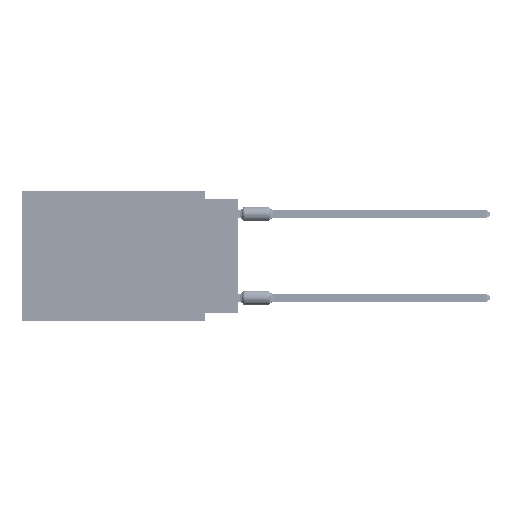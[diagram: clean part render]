
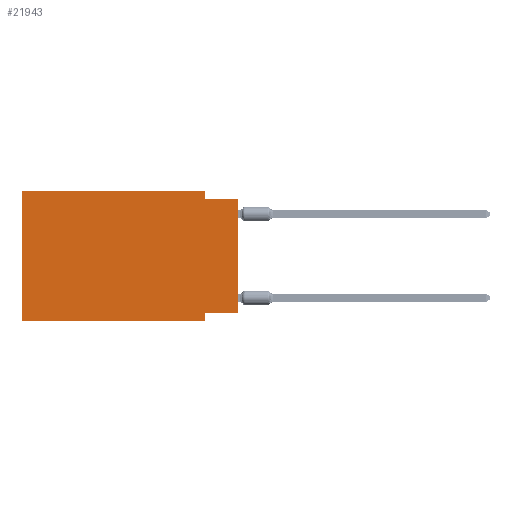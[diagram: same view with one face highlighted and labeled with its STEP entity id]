
A CAD part, left-side view. The second image highlights one B-rep face of the part: STEP entity #21943.
In plain terms, the highlighted planar face has unit normal (-1, 0, 0).
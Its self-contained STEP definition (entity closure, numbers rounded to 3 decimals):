
#1484 = LINE ( 'NONE', #72477, #11325 ) ;
#3203 = DIRECTION ( 'NONE',  ( 0., 0., 1. ) ) ;
#3818 = CARTESIAN_POINT ( 'NONE',  ( 0., 2.54, -9.271 ) ) ;
#4846 = VECTOR ( 'NONE', #40684, 1000. ) ;
#6662 = EDGE_LOOP ( 'NONE', ( #53667, #39461, #34079, #17401, #43383, #15683, #40412, #62274 ) ) ;
#9357 = DIRECTION ( 'NONE',  ( 0., -1., 0. ) ) ;
#11148 = EDGE_CURVE ( 'NONE', #65817, #14942, #81049, .T. ) ;
#11244 = VERTEX_POINT ( 'NONE', #76825 ) ;
#11325 = VECTOR ( 'NONE', #66577, 1000. ) ;
#13770 = CARTESIAN_POINT ( 'NONE',  ( 0., 16.383, 0. ) ) ;
#13896 = VERTEX_POINT ( 'NONE', #51735 ) ;
#14942 = VERTEX_POINT ( 'NONE', #24481 ) ;
#15283 = AXIS2_PLACEMENT_3D ( 'NONE', #20188, #45797, #71420 ) ;
#15683 = ORIENTED_EDGE ( 'NONE', *, *, #73483, .T. ) ;
#16409 = CARTESIAN_POINT ( 'NONE',  ( 0., 16.383, -9.906 ) ) ;
#16473 = CARTESIAN_POINT ( 'NONE',  ( 0., 0., -0.635 ) ) ;
#17401 = ORIENTED_EDGE ( 'NONE', *, *, #70530, .F. ) ;
#18033 = CARTESIAN_POINT ( 'NONE',  ( 0., 2.54, 0. ) ) ;
#18951 = FACE_OUTER_BOUND ( 'NONE', #6662, .T. ) ;
#20103 = VECTOR ( 'NONE', #43658, 1000. ) ;
#20188 = CARTESIAN_POINT ( 'NONE',  ( 0., 16.383, 0. ) ) ;
#21943 = ADVANCED_FACE ( 'NONE', ( #18951 ), #26496, .F. ) ;
#24481 = CARTESIAN_POINT ( 'NONE',  ( 0., 2.54, -0.635 ) ) ;
#24612 = VERTEX_POINT ( 'NONE', #16409 ) ;
#24982 = LINE ( 'NONE', #71158, #62120 ) ;
#25169 = LINE ( 'NONE', #13770, #52710 ) ;
#26496 = PLANE ( 'NONE',  #15283 ) ;
#28052 = VECTOR ( 'NONE', #3203, 1000. ) ;
#34079 = ORIENTED_EDGE ( 'NONE', *, *, #11148, .F. ) ;
#34270 = VERTEX_POINT ( 'NONE', #39317 ) ;
#34340 = LINE ( 'NONE', #66675, #28052 ) ;
#36101 = EDGE_CURVE ( 'NONE', #51958, #34270, #1484, .T. ) ;
#39230 = DIRECTION ( 'NONE',  ( 0., 1., 0. ) ) ;
#39317 = CARTESIAN_POINT ( 'NONE',  ( 0., 2.54, -9.906 ) ) ;
#39461 = ORIENTED_EDGE ( 'NONE', *, *, #48991, .F. ) ;
#39922 = EDGE_CURVE ( 'NONE', #24612, #13896, #46570, .T. ) ;
#40412 = ORIENTED_EDGE ( 'NONE', *, *, #36101, .F. ) ;
#40684 = DIRECTION ( 'NONE',  ( 0., 0., 1. ) ) ;
#41098 = CARTESIAN_POINT ( 'NONE',  ( 0., 16.383, 0. ) ) ;
#43383 = ORIENTED_EDGE ( 'NONE', *, *, #39922, .F. ) ;
#43652 = VECTOR ( 'NONE', #48009, 1000. ) ;
#43658 = DIRECTION ( 'NONE',  ( 0., 0., -1. ) ) ;
#44165 = EDGE_CURVE ( 'NONE', #78108, #11244, #34340, .T. ) ;
#45797 = DIRECTION ( 'NONE',  ( 1., 0., 0. ) ) ;
#46570 = LINE ( 'NONE', #41098, #4846 ) ;
#48009 = DIRECTION ( 'NONE',  ( 0., -1., 0. ) ) ;
#48821 = EDGE_CURVE ( 'NONE', #78108, #51958, #24982, .T. ) ;
#48991 = EDGE_CURVE ( 'NONE', #14942, #11244, #54295, .T. ) ;
#50773 = DIRECTION ( 'NONE',  ( 0., -1., 0. ) ) ;
#51735 = CARTESIAN_POINT ( 'NONE',  ( 0., 16.383, 0. ) ) ;
#51958 = VERTEX_POINT ( 'NONE', #3818 ) ;
#52710 = VECTOR ( 'NONE', #50773, 1000. ) ;
#53667 = ORIENTED_EDGE ( 'NONE', *, *, #44165, .T. ) ;
#54295 = LINE ( 'NONE', #16473, #63459 ) ;
#59797 = CARTESIAN_POINT ( 'NONE',  ( 0., 16.383, -9.906 ) ) ;
#62120 = VECTOR ( 'NONE', #39230, 1000. ) ;
#62274 = ORIENTED_EDGE ( 'NONE', *, *, #48821, .F. ) ;
#63459 = VECTOR ( 'NONE', #9357, 1000. ) ;
#65817 = VERTEX_POINT ( 'NONE', #78007 ) ;
#66577 = DIRECTION ( 'NONE',  ( 0., 0., -1. ) ) ;
#66675 = CARTESIAN_POINT ( 'NONE',  ( 0., 0., 0. ) ) ;
#70530 = EDGE_CURVE ( 'NONE', #13896, #65817, #25169, .T. ) ;
#71158 = CARTESIAN_POINT ( 'NONE',  ( 0., 0., -9.271 ) ) ;
#71420 = DIRECTION ( 'NONE',  ( 0., 0., -1. ) ) ;
#72477 = CARTESIAN_POINT ( 'NONE',  ( 0., 2.54, -9.906 ) ) ;
#73483 = EDGE_CURVE ( 'NONE', #24612, #34270, #80354, .T. ) ;
#75322 = CARTESIAN_POINT ( 'NONE',  ( 0., 0., -9.271 ) ) ;
#76825 = CARTESIAN_POINT ( 'NONE',  ( 0., 0., -0.635 ) ) ;
#78007 = CARTESIAN_POINT ( 'NONE',  ( 0., 2.54, 0. ) ) ;
#78108 = VERTEX_POINT ( 'NONE', #75322 ) ;
#80354 = LINE ( 'NONE', #59797, #43652 ) ;
#81049 = LINE ( 'NONE', #18033, #20103 ) ;
